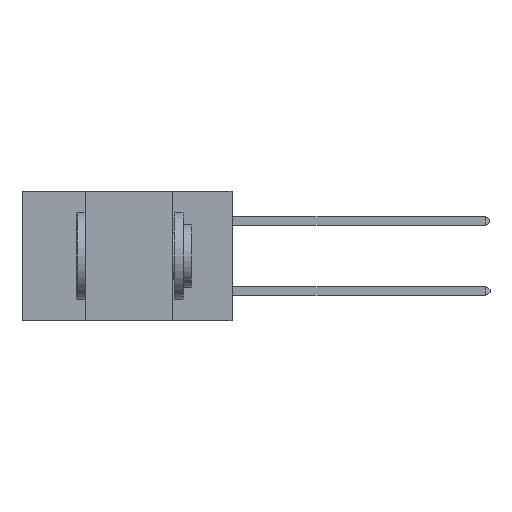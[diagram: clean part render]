
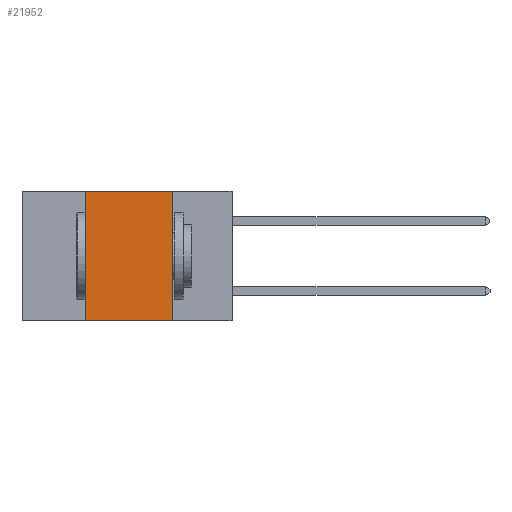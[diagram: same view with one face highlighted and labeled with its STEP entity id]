
A CAD part, left-side view. The second image highlights one B-rep face of the part: STEP entity #21952.
In plain terms, the highlighted planar face has unit normal (-1, 0, 0).
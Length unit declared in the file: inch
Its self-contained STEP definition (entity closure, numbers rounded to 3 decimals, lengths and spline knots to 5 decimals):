
#1941 = CARTESIAN_POINT ( 'NONE',  ( 0., 0.42, 0. ) ) ;
#2118 = EDGE_CURVE ( 'NONE', #17907, #10476, #18081, .T. ) ;
#2433 = ORIENTED_EDGE ( 'NONE', *, *, #17751, .F. ) ;
#2627 = VERTEX_POINT ( 'NONE', #11149 ) ;
#3031 = CARTESIAN_POINT ( 'NONE',  ( 0., 0.6, 0. ) ) ;
#3647 = VERTEX_POINT ( 'NONE', #19212 ) ;
#4106 = DIRECTION ( 'NONE',  ( 0., 0., -1. ) ) ;
#4270 = CARTESIAN_POINT ( 'NONE',  ( 0., 0.17, 0. ) ) ;
#4901 = DIRECTION ( 'NONE',  ( 0., 0., -1. ) ) ;
#6229 = LINE ( 'NONE', #18238, #15614 ) ;
#6581 = EDGE_CURVE ( 'NONE', #3647, #17907, #6229, .T. ) ;
#7011 = EDGE_CURVE ( 'NONE', #2627, #10476, #21702, .T. ) ;
#7738 = DIRECTION ( 'NONE',  ( 0., -1., 0. ) ) ;
#8302 = FACE_OUTER_BOUND ( 'NONE', #14339, .T. ) ;
#8476 = PLANE ( 'NONE',  #19700 ) ;
#9139 = CARTESIAN_POINT ( 'NONE',  ( 0., 0.17, -0.37 ) ) ;
#10476 = VERTEX_POINT ( 'NONE', #9139 ) ;
#11149 = CARTESIAN_POINT ( 'NONE',  ( 0., 0.42, -0.37 ) ) ;
#11503 = CARTESIAN_POINT ( 'NONE',  ( 0., 0.17, 0. ) ) ;
#11986 = LINE ( 'NONE', #1941, #16038 ) ;
#13494 = VECTOR ( 'NONE', #4106, 39.37008 ) ;
#14136 = DIRECTION ( 'NONE',  ( 0., -1., 0. ) ) ;
#14339 = EDGE_LOOP ( 'NONE', ( #18636, #16303, #2433, #15365 ) ) ;
#15365 = ORIENTED_EDGE ( 'NONE', *, *, #7011, .T. ) ;
#15530 = DIRECTION ( 'NONE',  ( 1., 0., 0. ) ) ;
#15614 = VECTOR ( 'NONE', #7738, 39.37008 ) ;
#16038 = VECTOR ( 'NONE', #19714, 39.37008 ) ;
#16303 = ORIENTED_EDGE ( 'NONE', *, *, #6581, .F. ) ;
#17549 = CARTESIAN_POINT ( 'NONE',  ( 0., 0.6, -0.37 ) ) ;
#17751 = EDGE_CURVE ( 'NONE', #2627, #3647, #11986, .T. ) ;
#17907 = VERTEX_POINT ( 'NONE', #11503 ) ;
#18081 = LINE ( 'NONE', #4270, #13494 ) ;
#18238 = CARTESIAN_POINT ( 'NONE',  ( 0., 0.6, 0. ) ) ;
#18636 = ORIENTED_EDGE ( 'NONE', *, *, #2118, .F. ) ;
#19212 = CARTESIAN_POINT ( 'NONE',  ( 0., 0.42, 0. ) ) ;
#19700 = AXIS2_PLACEMENT_3D ( 'NONE', #3031, #15530, #4901 ) ;
#19714 = DIRECTION ( 'NONE',  ( 0., 0., 1. ) ) ;
#20669 = VECTOR ( 'NONE', #14136, 39.37008 ) ;
#21702 = LINE ( 'NONE', #17549, #20669 ) ;
#21952 = ADVANCED_FACE ( 'NONE', ( #8302 ), #8476, .F. ) ;
